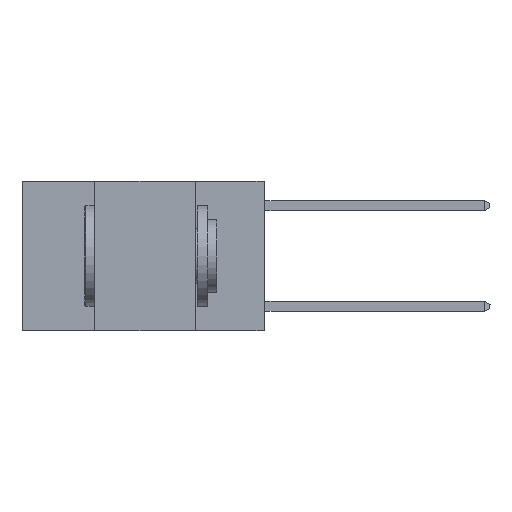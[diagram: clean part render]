
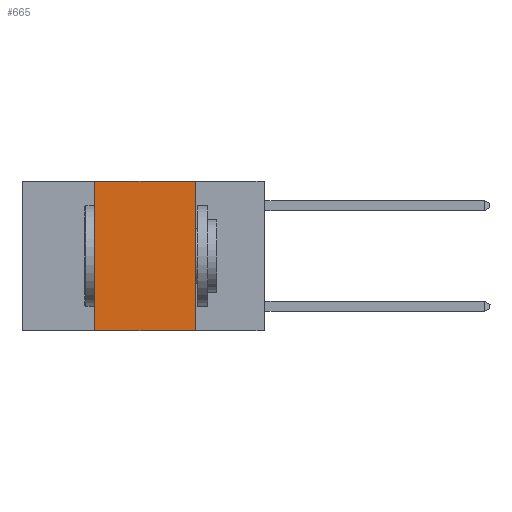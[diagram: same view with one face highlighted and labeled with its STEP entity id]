
A CAD part, left-side view. The second image highlights one B-rep face of the part: STEP entity #665.
In plain terms, the highlighted planar face has unit normal (-1, 0, 0).
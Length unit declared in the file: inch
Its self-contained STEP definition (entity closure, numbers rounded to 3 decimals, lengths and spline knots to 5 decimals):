
#665 = ADVANCED_FACE ( 'NONE', ( #11962 ), #21809, .F. ) ;
#673 = VERTEX_POINT ( 'NONE', #16480 ) ;
#1442 = VECTOR ( 'NONE', #17868, 39.37008 ) ;
#1924 = DIRECTION ( 'NONE',  ( 1., 0., 0. ) ) ;
#2011 = CARTESIAN_POINT ( 'NONE',  ( 0., 0.42, -0.37 ) ) ;
#2429 = VECTOR ( 'NONE', #12283, 39.37008 ) ;
#2595 = DIRECTION ( 'NONE',  ( 0., 0., -1. ) ) ;
#5496 = VERTEX_POINT ( 'NONE', #2011 ) ;
#7180 = CARTESIAN_POINT ( 'NONE',  ( 0., 0.17, 0. ) ) ;
#7366 = CARTESIAN_POINT ( 'NONE',  ( 0., 0.42, 0. ) ) ;
#8294 = EDGE_CURVE ( 'NONE', #23219, #13599, #14686, .T. ) ;
#9077 = VECTOR ( 'NONE', #9160, 39.37008 ) ;
#9160 = DIRECTION ( 'NONE',  ( 0., 0., 1. ) ) ;
#10182 = ORIENTED_EDGE ( 'NONE', *, *, #15402, .T. ) ;
#10822 = AXIS2_PLACEMENT_3D ( 'NONE', #16409, #1924, #14665 ) ;
#10992 = VECTOR ( 'NONE', #2595, 39.37008 ) ;
#11302 = ORIENTED_EDGE ( 'NONE', *, *, #19968, .F. ) ;
#11518 = EDGE_CURVE ( 'NONE', #673, #23219, #15992, .T. ) ;
#11962 = FACE_OUTER_BOUND ( 'NONE', #16428, .T. ) ;
#12283 = DIRECTION ( 'NONE',  ( 0., -1., 0. ) ) ;
#13599 = VERTEX_POINT ( 'NONE', #14728 ) ;
#13893 = LINE ( 'NONE', #7366, #9077 ) ;
#14665 = DIRECTION ( 'NONE',  ( 0., 0., -1. ) ) ;
#14686 = LINE ( 'NONE', #15323, #10992 ) ;
#14728 = CARTESIAN_POINT ( 'NONE',  ( 0., 0.17, -0.37 ) ) ;
#15323 = CARTESIAN_POINT ( 'NONE',  ( 0., 0.17, 0. ) ) ;
#15374 = ORIENTED_EDGE ( 'NONE', *, *, #8294, .F. ) ;
#15402 = EDGE_CURVE ( 'NONE', #5496, #13599, #16939, .T. ) ;
#15992 = LINE ( 'NONE', #16037, #1442 ) ;
#16037 = CARTESIAN_POINT ( 'NONE',  ( 0., 0.6, 0. ) ) ;
#16409 = CARTESIAN_POINT ( 'NONE',  ( 0., 0.6, 0. ) ) ;
#16428 = EDGE_LOOP ( 'NONE', ( #15374, #16492, #11302, #10182 ) ) ;
#16480 = CARTESIAN_POINT ( 'NONE',  ( 0., 0.42, 0. ) ) ;
#16492 = ORIENTED_EDGE ( 'NONE', *, *, #11518, .F. ) ;
#16939 = LINE ( 'NONE', #21347, #2429 ) ;
#17868 = DIRECTION ( 'NONE',  ( 0., -1., 0. ) ) ;
#19968 = EDGE_CURVE ( 'NONE', #5496, #673, #13893, .T. ) ;
#21347 = CARTESIAN_POINT ( 'NONE',  ( 0., 0.6, -0.37 ) ) ;
#21809 = PLANE ( 'NONE',  #10822 ) ;
#23219 = VERTEX_POINT ( 'NONE', #7180 ) ;
